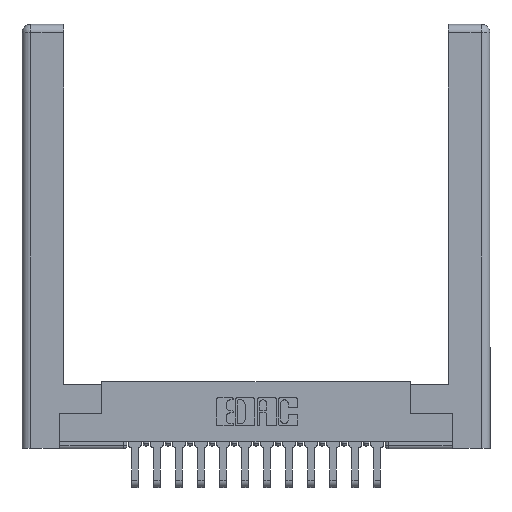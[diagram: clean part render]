
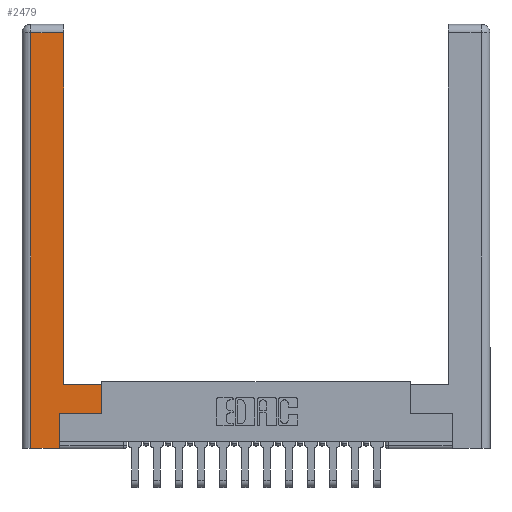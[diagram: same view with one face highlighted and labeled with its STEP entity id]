
A CAD part, top view. The second image highlights one B-rep face of the part: STEP entity #2479.
In plain terms, the highlighted planar face has unit normal (0, 0, 1).
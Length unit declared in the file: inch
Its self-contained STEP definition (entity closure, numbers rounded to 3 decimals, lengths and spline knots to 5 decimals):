
#422 = CARTESIAN_POINT ( 'NONE',  ( 0.0615, 0., 0. ) ) ;
#897 = CARTESIAN_POINT ( 'NONE',  ( 0.565, 0.245, 0. ) ) ;
#1383 = VERTEX_POINT ( 'NONE', #15565 ) ;
#1411 = EDGE_CURVE ( 'NONE', #8783, #18133, #5643, .T. ) ;
#1771 = ORIENTED_EDGE ( 'NONE', *, *, #8667, .T. ) ;
#2022 = DIRECTION ( 'NONE',  ( 1., 0., 0. ) ) ;
#2237 = VECTOR ( 'NONE', #2022, 39.37008 ) ;
#2305 = DIRECTION ( 'NONE',  ( 0., 0., -1. ) ) ;
#2399 = FACE_OUTER_BOUND ( 'NONE', #15071, .T. ) ;
#2479 = ADVANCED_FACE ( 'NONE', ( #2399 ), #17917, .F. ) ;
#2665 = CARTESIAN_POINT ( 'NONE',  ( 0.565, 0.45, 0. ) ) ;
#2855 = LINE ( 'NONE', #2665, #11684 ) ;
#3063 = DIRECTION ( 'NONE',  ( 0., 1., 0. ) ) ;
#3166 = LINE ( 'NONE', #8848, #18394 ) ;
#3454 = ORIENTED_EDGE ( 'NONE', *, *, #14221, .T. ) ;
#4135 = VERTEX_POINT ( 'NONE', #422 ) ;
#4339 = EDGE_CURVE ( 'NONE', #4135, #8783, #14832, .T. ) ;
#4434 = AXIS2_PLACEMENT_3D ( 'NONE', #5099, #2305, #8003 ) ;
#4866 = VECTOR ( 'NONE', #16303, 39.37008 ) ;
#4923 = DIRECTION ( 'NONE',  ( 0., -1., 0. ) ) ;
#5099 = CARTESIAN_POINT ( 'NONE',  ( 0., 0., 0. ) ) ;
#5155 = LINE ( 'NONE', #9455, #5971 ) ;
#5643 = LINE ( 'NONE', #7329, #9129 ) ;
#5789 = VERTEX_POINT ( 'NONE', #18353 ) ;
#5826 = CARTESIAN_POINT ( 'NONE',  ( 0.565, 0.45, 0. ) ) ;
#5858 = ORIENTED_EDGE ( 'NONE', *, *, #9525, .T. ) ;
#5971 = VECTOR ( 'NONE', #15165, 39.37008 ) ;
#6138 = EDGE_CURVE ( 'NONE', #1383, #8502, #5155, .T. ) ;
#6427 = ORIENTED_EDGE ( 'NONE', *, *, #6428, .T. ) ;
#6428 = EDGE_CURVE ( 'NONE', #5789, #1383, #17205, .T. ) ;
#7248 = DIRECTION ( 'NONE',  ( -1., 0., 0. ) ) ;
#7329 = CARTESIAN_POINT ( 'NONE',  ( 0.265, 0.245, 0. ) ) ;
#8003 = DIRECTION ( 'NONE',  ( -1., 0., 0. ) ) ;
#8356 = DIRECTION ( 'NONE',  ( 0., 1., 0. ) ) ;
#8502 = VERTEX_POINT ( 'NONE', #13052 ) ;
#8624 = VERTEX_POINT ( 'NONE', #5826 ) ;
#8667 = EDGE_CURVE ( 'NONE', #17685, #8624, #2855, .T. ) ;
#8783 = VERTEX_POINT ( 'NONE', #10409 ) ;
#8848 = CARTESIAN_POINT ( 'NONE',  ( 0.295, 0.45, 0. ) ) ;
#9129 = VECTOR ( 'NONE', #3063, 39.37008 ) ;
#9389 = LINE ( 'NONE', #897, #2237 ) ;
#9455 = CARTESIAN_POINT ( 'NONE',  ( 0.0615, 2.94, 0. ) ) ;
#9525 = EDGE_CURVE ( 'NONE', #8624, #5789, #3166, .T. ) ;
#10018 = ORIENTED_EDGE ( 'NONE', *, *, #1411, .T. ) ;
#10409 = CARTESIAN_POINT ( 'NONE',  ( 0.265, 0., 0. ) ) ;
#11684 = VECTOR ( 'NONE', #8356, 39.37008 ) ;
#11968 = CARTESIAN_POINT ( 'NONE',  ( 0.565, 0.245, 0. ) ) ;
#12058 = CARTESIAN_POINT ( 'NONE',  ( 0.0615, 0., 0. ) ) ;
#13052 = CARTESIAN_POINT ( 'NONE',  ( 0.0615, 2.94, 0. ) ) ;
#13469 = LINE ( 'NONE', #12058, #18402 ) ;
#13536 = CARTESIAN_POINT ( 'NONE',  ( 0.265, 0.245, 0. ) ) ;
#14221 = EDGE_CURVE ( 'NONE', #18133, #17685, #9389, .T. ) ;
#14412 = CARTESIAN_POINT ( 'NONE',  ( 0.295, 3., 0. ) ) ;
#14516 = ORIENTED_EDGE ( 'NONE', *, *, #17796, .T. ) ;
#14832 = LINE ( 'NONE', #16482, #4866 ) ;
#15071 = EDGE_LOOP ( 'NONE', ( #6427, #15159, #14516, #15681, #10018, #3454, #1771, #5858 ) ) ;
#15159 = ORIENTED_EDGE ( 'NONE', *, *, #6138, .T. ) ;
#15165 = DIRECTION ( 'NONE',  ( -1., 0., 0. ) ) ;
#15565 = CARTESIAN_POINT ( 'NONE',  ( 0.295, 2.94, 0. ) ) ;
#15681 = ORIENTED_EDGE ( 'NONE', *, *, #4339, .T. ) ;
#16133 = VECTOR ( 'NONE', #17308, 39.37008 ) ;
#16303 = DIRECTION ( 'NONE',  ( 1., 0., 0. ) ) ;
#16482 = CARTESIAN_POINT ( 'NONE',  ( 0.265, 0., 0. ) ) ;
#17205 = LINE ( 'NONE', #14412, #16133 ) ;
#17308 = DIRECTION ( 'NONE',  ( 0., 1., 0. ) ) ;
#17685 = VERTEX_POINT ( 'NONE', #11968 ) ;
#17796 = EDGE_CURVE ( 'NONE', #8502, #4135, #13469, .T. ) ;
#17917 = PLANE ( 'NONE',  #4434 ) ;
#18133 = VERTEX_POINT ( 'NONE', #13536 ) ;
#18353 = CARTESIAN_POINT ( 'NONE',  ( 0.295, 0.45, 0. ) ) ;
#18394 = VECTOR ( 'NONE', #7248, 39.37008 ) ;
#18402 = VECTOR ( 'NONE', #4923, 39.37008 ) ;
